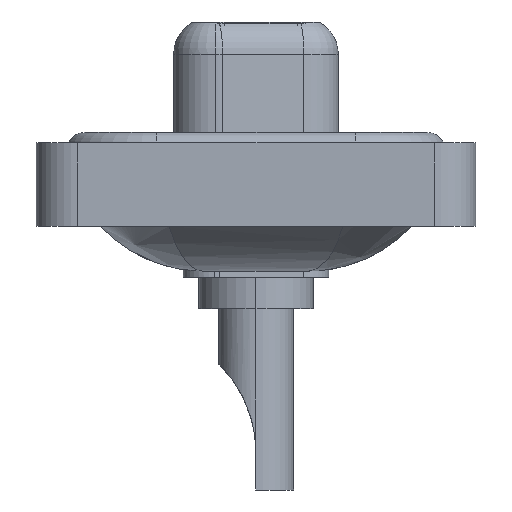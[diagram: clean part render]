
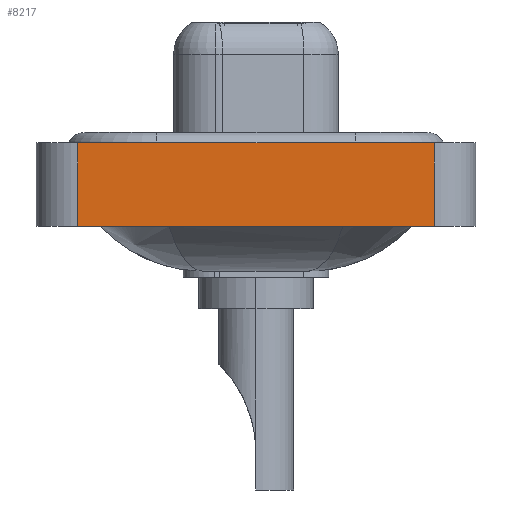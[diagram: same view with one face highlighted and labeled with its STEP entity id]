
A CAD part, left-side view. The second image highlights one B-rep face of the part: STEP entity #8217.
In plain terms, the highlighted planar face has unit normal (-1, 0, 0).
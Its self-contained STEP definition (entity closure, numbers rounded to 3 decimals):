
#628 = ORIENTED_EDGE ( 'NONE', *, *, #10502, .T. ) ;
#1005 = VECTOR ( 'NONE', #3799, 1000. ) ;
#1755 = VERTEX_POINT ( 'NONE', #13256 ) ;
#2186 = DIRECTION ( 'NONE',  ( -1., 0., 0. ) ) ;
#2229 = DIRECTION ( 'NONE',  ( 0., -1., 0. ) ) ;
#2573 = CARTESIAN_POINT ( 'NONE',  ( -7.3, 8.55, -3.6 ) ) ;
#2692 = CARTESIAN_POINT ( 'NONE',  ( -7.3, -8.55, -3.6 ) ) ;
#3799 = DIRECTION ( 'NONE',  ( 0., 0., 1. ) ) ;
#3955 = DIRECTION ( 'NONE',  ( 0., -1., 0. ) ) ;
#4562 = FACE_OUTER_BOUND ( 'NONE', #10517, .T. ) ;
#4841 = CARTESIAN_POINT ( 'NONE',  ( -7.3, -8.55, -3.6 ) ) ;
#6020 = DIRECTION ( 'NONE',  ( 0., 0., 1. ) ) ;
#6770 = CARTESIAN_POINT ( 'NONE',  ( -7.3, 8.55, 0.4 ) ) ;
#6809 = DIRECTION ( 'NONE',  ( 0., 0., 1. ) ) ;
#7780 = LINE ( 'NONE', #2573, #1005 ) ;
#8217 = ADVANCED_FACE ( 'NONE', ( #4562 ), #8369, .T. ) ;
#8369 = PLANE ( 'NONE',  #13355 ) ;
#9297 = EDGE_CURVE ( 'NONE', #1755, #12613, #14709, .T. ) ;
#10502 = EDGE_CURVE ( 'NONE', #12613, #11661, #14165, .T. ) ;
#10517 = EDGE_LOOP ( 'NONE', ( #628, #14557, #16042, #14134 ) ) ;
#10686 = VECTOR ( 'NONE', #3955, 1000. ) ;
#11090 = VECTOR ( 'NONE', #2229, 1000. ) ;
#11661 = VERTEX_POINT ( 'NONE', #13279 ) ;
#11748 = EDGE_CURVE ( 'NONE', #12792, #11661, #12597, .T. ) ;
#12597 = LINE ( 'NONE', #14981, #10686 ) ;
#12613 = VERTEX_POINT ( 'NONE', #2692 ) ;
#12792 = VERTEX_POINT ( 'NONE', #6770 ) ;
#12930 = CARTESIAN_POINT ( 'NONE',  ( -7.3, -8.55, -3.6 ) ) ;
#13256 = CARTESIAN_POINT ( 'NONE',  ( -7.3, 8.55, -3.6 ) ) ;
#13279 = CARTESIAN_POINT ( 'NONE',  ( -7.3, -8.55, 0.4 ) ) ;
#13355 = AXIS2_PLACEMENT_3D ( 'NONE', #13364, #2186, #6020 ) ;
#13364 = CARTESIAN_POINT ( 'NONE',  ( -7.3, -8.55, -3.6 ) ) ;
#13475 = VECTOR ( 'NONE', #6809, 1000. ) ;
#14134 = ORIENTED_EDGE ( 'NONE', *, *, #9297, .T. ) ;
#14165 = LINE ( 'NONE', #12930, #13475 ) ;
#14557 = ORIENTED_EDGE ( 'NONE', *, *, #11748, .F. ) ;
#14620 = EDGE_CURVE ( 'NONE', #1755, #12792, #7780, .T. ) ;
#14709 = LINE ( 'NONE', #4841, #11090 ) ;
#14981 = CARTESIAN_POINT ( 'NONE',  ( -7.3, -8.55, 0.4 ) ) ;
#16042 = ORIENTED_EDGE ( 'NONE', *, *, #14620, .F. ) ;
